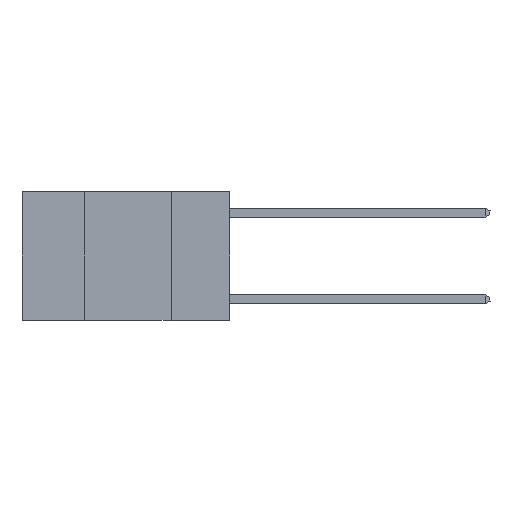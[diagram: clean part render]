
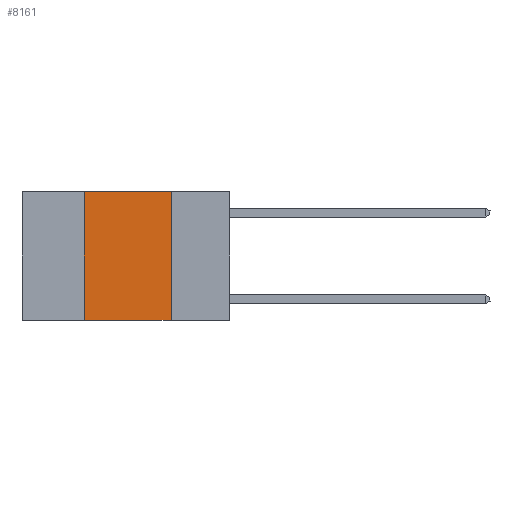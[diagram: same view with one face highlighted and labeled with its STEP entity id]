
A CAD part, left-side view. The second image highlights one B-rep face of the part: STEP entity #8161.
In plain terms, the highlighted planar face has unit normal (-1, 0, 0).
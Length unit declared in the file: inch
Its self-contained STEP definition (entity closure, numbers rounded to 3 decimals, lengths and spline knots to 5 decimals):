
#690 = PLANE ( 'NONE',  #6087 ) ;
#835 = LINE ( 'NONE', #7897, #6557 ) ;
#988 = VERTEX_POINT ( 'NONE', #22885 ) ;
#1036 = CARTESIAN_POINT ( 'NONE',  ( 0., 0.42, 0. ) ) ;
#1484 = DIRECTION ( 'NONE',  ( 0., -1., 0. ) ) ;
#2155 = CARTESIAN_POINT ( 'NONE',  ( 0., 0.17, 0. ) ) ;
#3288 = VECTOR ( 'NONE', #1484, 39.37008 ) ;
#3913 = LINE ( 'NONE', #9781, #13853 ) ;
#3933 = CARTESIAN_POINT ( 'NONE',  ( 0., 0.42, -0.37 ) ) ;
#4098 = VERTEX_POINT ( 'NONE', #2155 ) ;
#4353 = ORIENTED_EDGE ( 'NONE', *, *, #23212, .F. ) ;
#5036 = DIRECTION ( 'NONE',  ( 1., 0., 0. ) ) ;
#5469 = EDGE_LOOP ( 'NONE', ( #18985, #14995, #4353, #9830 ) ) ;
#6087 = AXIS2_PLACEMENT_3D ( 'NONE', #17737, #5036, #19888 ) ;
#6557 = VECTOR ( 'NONE', #22784, 39.37008 ) ;
#7897 = CARTESIAN_POINT ( 'NONE',  ( 0., 0.17, 0. ) ) ;
#8161 = ADVANCED_FACE ( 'NONE', ( #23978 ), #690, .F. ) ;
#8638 = LINE ( 'NONE', #17803, #19927 ) ;
#9778 = VERTEX_POINT ( 'NONE', #3933 ) ;
#9781 = CARTESIAN_POINT ( 'NONE',  ( 0., 0.6, -0.37 ) ) ;
#9830 = ORIENTED_EDGE ( 'NONE', *, *, #24628, .T. ) ;
#13853 = VECTOR ( 'NONE', #24664, 39.37008 ) ;
#14201 = CARTESIAN_POINT ( 'NONE',  ( 0., 0.6, 0. ) ) ;
#14995 = ORIENTED_EDGE ( 'NONE', *, *, #17649, .F. ) ;
#15566 = VERTEX_POINT ( 'NONE', #1036 ) ;
#17649 = EDGE_CURVE ( 'NONE', #15566, #4098, #20252, .T. ) ;
#17737 = CARTESIAN_POINT ( 'NONE',  ( 0., 0.6, 0. ) ) ;
#17803 = CARTESIAN_POINT ( 'NONE',  ( 0., 0.42, 0. ) ) ;
#18887 = EDGE_CURVE ( 'NONE', #4098, #988, #835, .T. ) ;
#18985 = ORIENTED_EDGE ( 'NONE', *, *, #18887, .F. ) ;
#19888 = DIRECTION ( 'NONE',  ( 0., 0., -1. ) ) ;
#19927 = VECTOR ( 'NONE', #26292, 39.37008 ) ;
#20252 = LINE ( 'NONE', #14201, #3288 ) ;
#22784 = DIRECTION ( 'NONE',  ( 0., 0., -1. ) ) ;
#22885 = CARTESIAN_POINT ( 'NONE',  ( 0., 0.17, -0.37 ) ) ;
#23212 = EDGE_CURVE ( 'NONE', #9778, #15566, #8638, .T. ) ;
#23978 = FACE_OUTER_BOUND ( 'NONE', #5469, .T. ) ;
#24628 = EDGE_CURVE ( 'NONE', #9778, #988, #3913, .T. ) ;
#24664 = DIRECTION ( 'NONE',  ( 0., -1., 0. ) ) ;
#26292 = DIRECTION ( 'NONE',  ( 0., 0., 1. ) ) ;
